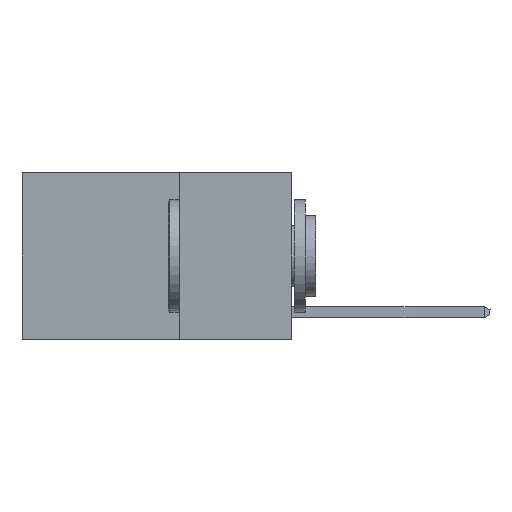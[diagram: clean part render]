
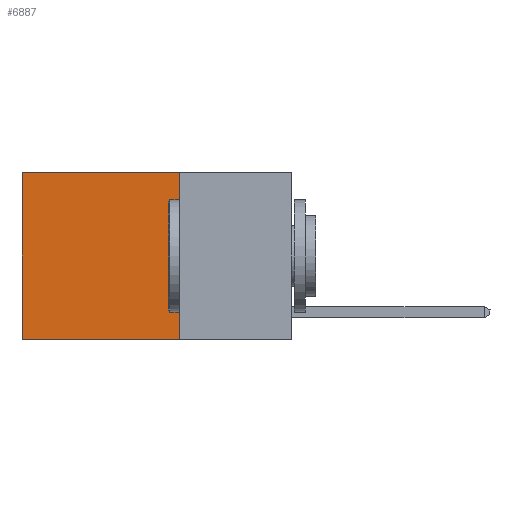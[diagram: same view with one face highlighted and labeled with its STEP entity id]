
A CAD part, left-side view. The second image highlights one B-rep face of the part: STEP entity #6887.
In plain terms, the highlighted planar face has unit normal (-1, 0, 0).
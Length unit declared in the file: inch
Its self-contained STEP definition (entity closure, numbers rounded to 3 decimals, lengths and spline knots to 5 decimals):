
#303 = DIRECTION ( 'NONE',  ( 0., 1., 0. ) ) ;
#643 = AXIS2_PLACEMENT_3D ( 'NONE', #5874, #12824, #28709 ) ;
#1068 = VECTOR ( 'NONE', #25447, 39.37008 ) ;
#1571 = VECTOR ( 'NONE', #303, 39.37008 ) ;
#2382 = VERTEX_POINT ( 'NONE', #29536 ) ;
#2770 = CARTESIAN_POINT ( 'NONE',  ( 0.2625, 0.25, 0. ) ) ;
#5874 = CARTESIAN_POINT ( 'NONE',  ( 0.2625, 0.25, 0. ) ) ;
#6352 = LINE ( 'NONE', #13672, #23891 ) ;
#6887 = ADVANCED_FACE ( 'NONE', ( #11602 ), #26432, .F. ) ;
#7363 = VERTEX_POINT ( 'NONE', #15875 ) ;
#7997 = DIRECTION ( 'NONE',  ( 0., 0., -1. ) ) ;
#9052 = DIRECTION ( 'NONE',  ( 0., 0., -1. ) ) ;
#11602 = FACE_OUTER_BOUND ( 'NONE', #19762, .T. ) ;
#11862 = CARTESIAN_POINT ( 'NONE',  ( 0.2625, 0.25, -0.37 ) ) ;
#12824 = DIRECTION ( 'NONE',  ( 1., 0., 0. ) ) ;
#13672 = CARTESIAN_POINT ( 'NONE',  ( 0.2625, 0.25, 0. ) ) ;
#14029 = CARTESIAN_POINT ( 'NONE',  ( 0.2625, 0.25, 0. ) ) ;
#15875 = CARTESIAN_POINT ( 'NONE',  ( 0.2625, 0.25, -0.37 ) ) ;
#16455 = ORIENTED_EDGE ( 'NONE', *, *, #19501, .F. ) ;
#18432 = EDGE_CURVE ( 'NONE', #22814, #27731, #19436, .T. ) ;
#18726 = ORIENTED_EDGE ( 'NONE', *, *, #18432, .T. ) ;
#18989 = VECTOR ( 'NONE', #7997, 39.37008 ) ;
#19436 = LINE ( 'NONE', #14029, #1068 ) ;
#19501 = EDGE_CURVE ( 'NONE', #22814, #7363, #6352, .T. ) ;
#19762 = EDGE_LOOP ( 'NONE', ( #27613, #27016, #16455, #18726 ) ) ;
#20894 = EDGE_CURVE ( 'NONE', #7363, #2382, #25949, .T. ) ;
#21704 = CARTESIAN_POINT ( 'NONE',  ( 0.2625, 0.6, 0. ) ) ;
#22814 = VERTEX_POINT ( 'NONE', #2770 ) ;
#23891 = VECTOR ( 'NONE', #9052, 39.37008 ) ;
#24202 = EDGE_CURVE ( 'NONE', #27731, #2382, #25023, .T. ) ;
#25023 = LINE ( 'NONE', #21704, #18989 ) ;
#25447 = DIRECTION ( 'NONE',  ( 0., 1., 0. ) ) ;
#25949 = LINE ( 'NONE', #11862, #1571 ) ;
#26052 = CARTESIAN_POINT ( 'NONE',  ( 0.2625, 0.6, 0. ) ) ;
#26432 = PLANE ( 'NONE',  #643 ) ;
#27016 = ORIENTED_EDGE ( 'NONE', *, *, #20894, .F. ) ;
#27613 = ORIENTED_EDGE ( 'NONE', *, *, #24202, .T. ) ;
#27731 = VERTEX_POINT ( 'NONE', #26052 ) ;
#28709 = DIRECTION ( 'NONE',  ( 0., 0., -1. ) ) ;
#29536 = CARTESIAN_POINT ( 'NONE',  ( 0.2625, 0.6, -0.37 ) ) ;
